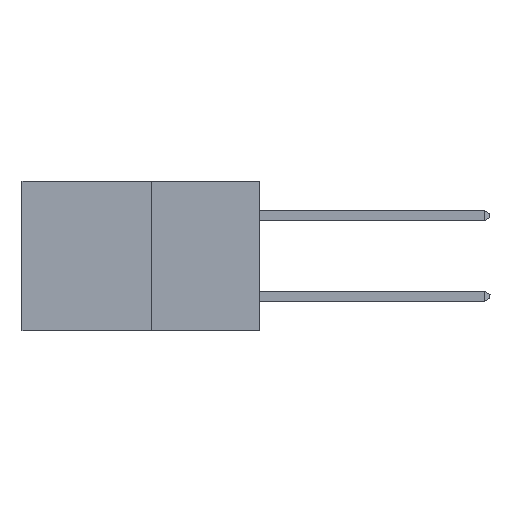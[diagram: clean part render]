
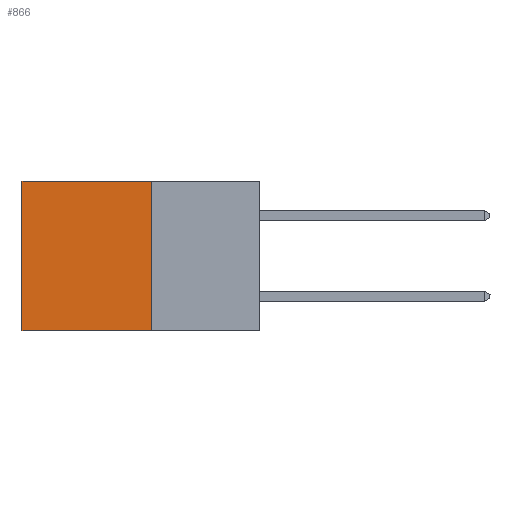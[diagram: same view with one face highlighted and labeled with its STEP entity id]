
A CAD part, left-side view. The second image highlights one B-rep face of the part: STEP entity #866.
In plain terms, the highlighted planar face has unit normal (-1, 0, 0).
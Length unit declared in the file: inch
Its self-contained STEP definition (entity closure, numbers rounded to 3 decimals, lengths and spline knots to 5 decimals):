
#705 = EDGE_CURVE ( 'NONE', #4451, #2777, #7889, .T. ) ;
#866 = ADVANCED_FACE ( 'NONE', ( #8226 ), #9130, .F. ) ;
#936 = CARTESIAN_POINT ( 'NONE',  ( 0.277, 0.59, -0.37 ) ) ;
#966 = VECTOR ( 'NONE', #1205, 39.37008 ) ;
#1205 = DIRECTION ( 'NONE',  ( 0., 1., 0. ) ) ;
#1572 = ORIENTED_EDGE ( 'NONE', *, *, #8996, .T. ) ;
#1853 = ORIENTED_EDGE ( 'NONE', *, *, #8334, .F. ) ;
#2015 = EDGE_LOOP ( 'NONE', ( #1572, #2790, #1853, #3178 ) ) ;
#2290 = VECTOR ( 'NONE', #9954, 39.37008 ) ;
#2530 = VERTEX_POINT ( 'NONE', #936 ) ;
#2777 = VERTEX_POINT ( 'NONE', #6764 ) ;
#2790 = ORIENTED_EDGE ( 'NONE', *, *, #7697, .F. ) ;
#3178 = ORIENTED_EDGE ( 'NONE', *, *, #705, .T. ) ;
#3933 = CARTESIAN_POINT ( 'NONE',  ( 0.277, 0.59, -0.37 ) ) ;
#4451 = VERTEX_POINT ( 'NONE', #4496 ) ;
#4496 = CARTESIAN_POINT ( 'NONE',  ( 0.277, 0.27, 0. ) ) ;
#4597 = LINE ( 'NONE', #5745, #966 ) ;
#4950 = AXIS2_PLACEMENT_3D ( 'NONE', #7382, #9157, #6291 ) ;
#5394 = VECTOR ( 'NONE', #5608, 39.37008 ) ;
#5608 = DIRECTION ( 'NONE',  ( 0., 0., -1. ) ) ;
#5745 = CARTESIAN_POINT ( 'NONE',  ( 0.277, 0.27, -0.37 ) ) ;
#6212 = DIRECTION ( 'NONE',  ( 0., 0., -1. ) ) ;
#6291 = DIRECTION ( 'NONE',  ( 0., 0., -1. ) ) ;
#6428 = CARTESIAN_POINT ( 'NONE',  ( 0.277, 0.27, -0.37 ) ) ;
#6570 = VECTOR ( 'NONE', #6212, 39.37008 ) ;
#6764 = CARTESIAN_POINT ( 'NONE',  ( 0.277, 0.59, 0. ) ) ;
#7382 = CARTESIAN_POINT ( 'NONE',  ( 0.277, 0.27, -0.37 ) ) ;
#7450 = LINE ( 'NONE', #7878, #5394 ) ;
#7697 = EDGE_CURVE ( 'NONE', #8380, #2530, #4597, .T. ) ;
#7878 = CARTESIAN_POINT ( 'NONE',  ( 0.277, 0.27, -0.37 ) ) ;
#7889 = LINE ( 'NONE', #8250, #2290 ) ;
#8226 = FACE_OUTER_BOUND ( 'NONE', #2015, .T. ) ;
#8250 = CARTESIAN_POINT ( 'NONE',  ( 0.277, 0.27, 0. ) ) ;
#8334 = EDGE_CURVE ( 'NONE', #4451, #8380, #7450, .T. ) ;
#8380 = VERTEX_POINT ( 'NONE', #6428 ) ;
#8823 = LINE ( 'NONE', #3933, #6570 ) ;
#8996 = EDGE_CURVE ( 'NONE', #2777, #2530, #8823, .T. ) ;
#9130 = PLANE ( 'NONE',  #4950 ) ;
#9157 = DIRECTION ( 'NONE',  ( 1., 0., 0. ) ) ;
#9954 = DIRECTION ( 'NONE',  ( 0., 1., 0. ) ) ;
